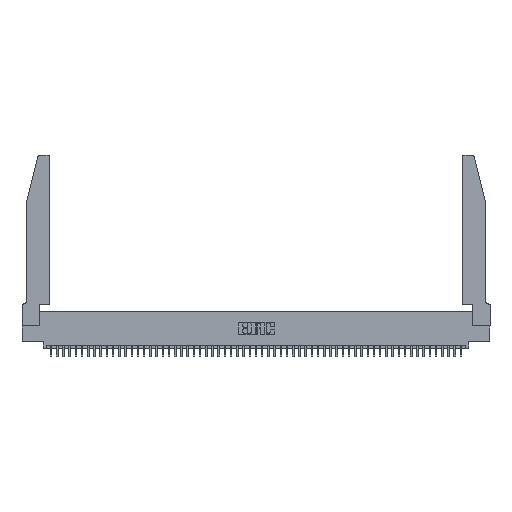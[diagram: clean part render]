
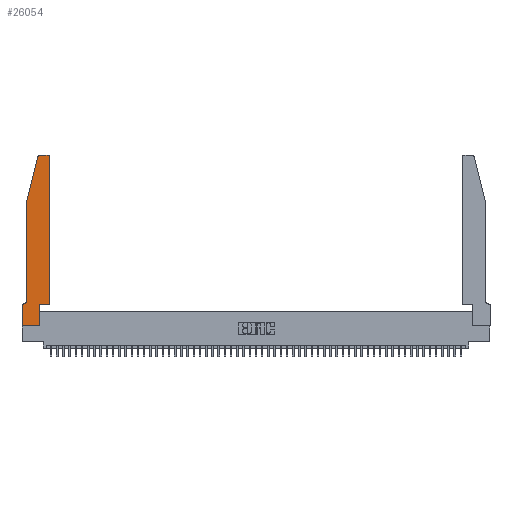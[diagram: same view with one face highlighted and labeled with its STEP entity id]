
A CAD part, top view. The second image highlights one B-rep face of the part: STEP entity #26054.
In plain terms, the highlighted planar face has unit normal (0, 0, 1).
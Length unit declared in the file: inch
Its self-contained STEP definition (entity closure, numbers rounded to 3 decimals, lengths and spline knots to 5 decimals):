
#80 = DIRECTION ( 'NONE',  ( -0.239, -0.971, 0. ) ) ;
#1285 = LINE ( 'NONE', #7923, #32132 ) ;
#2013 = VECTOR ( 'NONE', #22074, 39.37008 ) ;
#2189 = DIRECTION ( 'NONE',  ( 0., -1., 0. ) ) ;
#2411 = EDGE_CURVE ( 'NONE', #33707, #27534, #46149, .T. ) ;
#3343 = ORIENTED_EDGE ( 'NONE', *, *, #42050, .T. ) ;
#3954 = PLANE ( 'NONE',  #43781 ) ;
#4648 = VECTOR ( 'NONE', #40285, 39.37008 ) ;
#7164 = CARTESIAN_POINT ( 'NONE',  ( 0.4205, 2.75, 0.37 ) ) ;
#7188 = DIRECTION ( 'NONE',  ( -1., 0., 0. ) ) ;
#7272 = EDGE_CURVE ( 'NONE', #36602, #25376, #47217, .T. ) ;
#7923 = CARTESIAN_POINT ( 'NONE',  ( 0.0755, 2., 0.37 ) ) ;
#8223 = DIRECTION ( 'NONE',  ( 0., 0., 1. ) ) ;
#8595 = VECTOR ( 'NONE', #7188, 39.37008 ) ;
#8725 = CARTESIAN_POINT ( 'NONE',  ( 0.0755, 0.42, 0.37 ) ) ;
#8786 = ORIENTED_EDGE ( 'NONE', *, *, #10616, .T. ) ;
#9351 = CIRCLE ( 'NONE', #10889, 0.07 ) ;
#9997 = VERTEX_POINT ( 'NONE', #46770 ) ;
#10616 = EDGE_CURVE ( 'NONE', #41624, #33707, #24102, .T. ) ;
#10621 = CARTESIAN_POINT ( 'NONE',  ( 0.4205, 2.72, 0.37 ) ) ;
#10649 = LINE ( 'NONE', #51218, #2013 ) ;
#10889 = AXIS2_PLACEMENT_3D ( 'NONE', #20049, #49221, #24248 ) ;
#11586 = VECTOR ( 'NONE', #2189, 39.37008 ) ;
#12563 = CARTESIAN_POINT ( 'NONE',  ( 0.284, 2.72, 0.37 ) ) ;
#13432 = VERTEX_POINT ( 'NONE', #27031 ) ;
#13796 = CIRCLE ( 'NONE', #37245, 0.03 ) ;
#14361 = VERTEX_POINT ( 'NONE', #7164 ) ;
#14839 = DIRECTION ( 'NONE',  ( 1., 0., 0. ) ) ;
#14932 = ORIENTED_EDGE ( 'NONE', *, *, #53818, .T. ) ;
#15487 = CARTESIAN_POINT ( 'NONE',  ( 0.2605, 2.75, 0.37 ) ) ;
#16753 = DIRECTION ( 'NONE',  ( 1., 0., 0. ) ) ;
#17225 = EDGE_CURVE ( 'NONE', #37351, #13432, #10649, .T. ) ;
#17402 = CARTESIAN_POINT ( 'NONE',  ( 0.0755, 0.35, 0.37 ) ) ;
#17711 = CARTESIAN_POINT ( 'NONE',  ( 0.0755, 2., 0.37 ) ) ;
#17847 = CARTESIAN_POINT ( 'NONE',  ( 0., 0., 0.37 ) ) ;
#19603 = ORIENTED_EDGE ( 'NONE', *, *, #37053, .T. ) ;
#20049 = CARTESIAN_POINT ( 'NONE',  ( 0.0055, 0.42, 0.37 ) ) ;
#20564 = DIRECTION ( 'NONE',  ( 0., -1., 0. ) ) ;
#21525 = ORIENTED_EDGE ( 'NONE', *, *, #23824, .T. ) ;
#21677 = VERTEX_POINT ( 'NONE', #17711 ) ;
#22074 = DIRECTION ( 'NONE',  ( 0., 1., 0. ) ) ;
#23403 = EDGE_CURVE ( 'NONE', #35899, #21677, #38774, .T. ) ;
#23824 = EDGE_CURVE ( 'NONE', #41451, #41624, #9351, .T. ) ;
#24102 = LINE ( 'NONE', #17402, #35201 ) ;
#24248 = DIRECTION ( 'NONE',  ( -1., 0., 0. ) ) ;
#25140 = CARTESIAN_POINT ( 'NONE',  ( 0.4505, 2.72, 0.37 ) ) ;
#25202 = EDGE_CURVE ( 'NONE', #14361, #9997, #41942, .T. ) ;
#25228 = CARTESIAN_POINT ( 'NONE',  ( 0.0755, 2., 0.37 ) ) ;
#25376 = VERTEX_POINT ( 'NONE', #25140 ) ;
#26054 = ADVANCED_FACE ( 'NONE', ( #41807 ), #3954, .T. ) ;
#26783 = EDGE_LOOP ( 'NONE', ( #48512, #3343, #39162, #34583, #21525, #8786, #38417, #19603, #40739, #46735, #39528, #14932 ) ) ;
#27031 = CARTESIAN_POINT ( 'NONE',  ( 0.2865, 0.35, 0.37 ) ) ;
#27534 = VERTEX_POINT ( 'NONE', #35131 ) ;
#28405 = CARTESIAN_POINT ( 'NONE',  ( 0.2865, 0., 0.37 ) ) ;
#29103 = CARTESIAN_POINT ( 'NONE',  ( 0., 0.35, 0.37 ) ) ;
#29888 = VECTOR ( 'NONE', #42821, 39.37008 ) ;
#31531 = CARTESIAN_POINT ( 'NONE',  ( 0., 0., 0.37 ) ) ;
#32106 = CARTESIAN_POINT ( 'NONE',  ( 0.4505, 0.35, 0.37 ) ) ;
#32132 = VECTOR ( 'NONE', #20564, 39.37008 ) ;
#33707 = VERTEX_POINT ( 'NONE', #44128 ) ;
#34459 = EDGE_CURVE ( 'NONE', #21677, #41451, #1285, .T. ) ;
#34583 = ORIENTED_EDGE ( 'NONE', *, *, #34459, .T. ) ;
#35131 = CARTESIAN_POINT ( 'NONE',  ( 0., 0., 0.37 ) ) ;
#35201 = VECTOR ( 'NONE', #38172, 39.37008 ) ;
#35899 = VERTEX_POINT ( 'NONE', #45926 ) ;
#36188 = VECTOR ( 'NONE', #41818, 39.37008 ) ;
#36602 = VERTEX_POINT ( 'NONE', #41700 ) ;
#36762 = LINE ( 'NONE', #32106, #4648 ) ;
#37053 = EDGE_CURVE ( 'NONE', #27534, #37351, #39641, .T. ) ;
#37245 = AXIS2_PLACEMENT_3D ( 'NONE', #10621, #39804, #14839 ) ;
#37351 = VERTEX_POINT ( 'NONE', #28405 ) ;
#37463 = DIRECTION ( 'NONE',  ( 1., 0., 0. ) ) ;
#37606 = CARTESIAN_POINT ( 'NONE',  ( 0.4505, 0.35, 0.37 ) ) ;
#37879 = CIRCLE ( 'NONE', #51557, 0.03 ) ;
#38172 = DIRECTION ( 'NONE',  ( -1., 0., 0. ) ) ;
#38417 = ORIENTED_EDGE ( 'NONE', *, *, #2411, .T. ) ;
#38774 = LINE ( 'NONE', #25228, #49855 ) ;
#39162 = ORIENTED_EDGE ( 'NONE', *, *, #23403, .T. ) ;
#39528 = ORIENTED_EDGE ( 'NONE', *, *, #7272, .T. ) ;
#39641 = LINE ( 'NONE', #17847, #29888 ) ;
#39804 = DIRECTION ( 'NONE',  ( 0., 0., 1. ) ) ;
#40285 = DIRECTION ( 'NONE',  ( 1., 0., 0. ) ) ;
#40739 = ORIENTED_EDGE ( 'NONE', *, *, #17225, .T. ) ;
#41451 = VERTEX_POINT ( 'NONE', #8725 ) ;
#41624 = VERTEX_POINT ( 'NONE', #43030 ) ;
#41700 = CARTESIAN_POINT ( 'NONE',  ( 0.4505, 0.35, 0.37 ) ) ;
#41735 = DIRECTION ( 'NONE',  ( 0., 0., 1. ) ) ;
#41807 = FACE_OUTER_BOUND ( 'NONE', #26783, .T. ) ;
#41818 = DIRECTION ( 'NONE',  ( 0., 1., 0. ) ) ;
#41942 = LINE ( 'NONE', #15487, #8595 ) ;
#42050 = EDGE_CURVE ( 'NONE', #9997, #35899, #37879, .T. ) ;
#42821 = DIRECTION ( 'NONE',  ( 1., 0., 0. ) ) ;
#43030 = CARTESIAN_POINT ( 'NONE',  ( 0.0055, 0.35, 0.37 ) ) ;
#43781 = AXIS2_PLACEMENT_3D ( 'NONE', #29103, #8223, #37463 ) ;
#44128 = CARTESIAN_POINT ( 'NONE',  ( 0., 0.35, 0.37 ) ) ;
#45926 = CARTESIAN_POINT ( 'NONE',  ( 0.25487, 2.72718, 0.37 ) ) ;
#46149 = LINE ( 'NONE', #31531, #11586 ) ;
#46735 = ORIENTED_EDGE ( 'NONE', *, *, #52634, .T. ) ;
#46770 = CARTESIAN_POINT ( 'NONE',  ( 0.284, 2.75, 0.37 ) ) ;
#47217 = LINE ( 'NONE', #37606, #36188 ) ;
#48512 = ORIENTED_EDGE ( 'NONE', *, *, #25202, .T. ) ;
#49221 = DIRECTION ( 'NONE',  ( 0., 0., -1. ) ) ;
#49855 = VECTOR ( 'NONE', #80, 39.37008 ) ;
#51218 = CARTESIAN_POINT ( 'NONE',  ( 0.2865, 0.35, 0.37 ) ) ;
#51557 = AXIS2_PLACEMENT_3D ( 'NONE', #12563, #41735, #16753 ) ;
#52634 = EDGE_CURVE ( 'NONE', #13432, #36602, #36762, .T. ) ;
#53818 = EDGE_CURVE ( 'NONE', #25376, #14361, #13796, .T. ) ;
